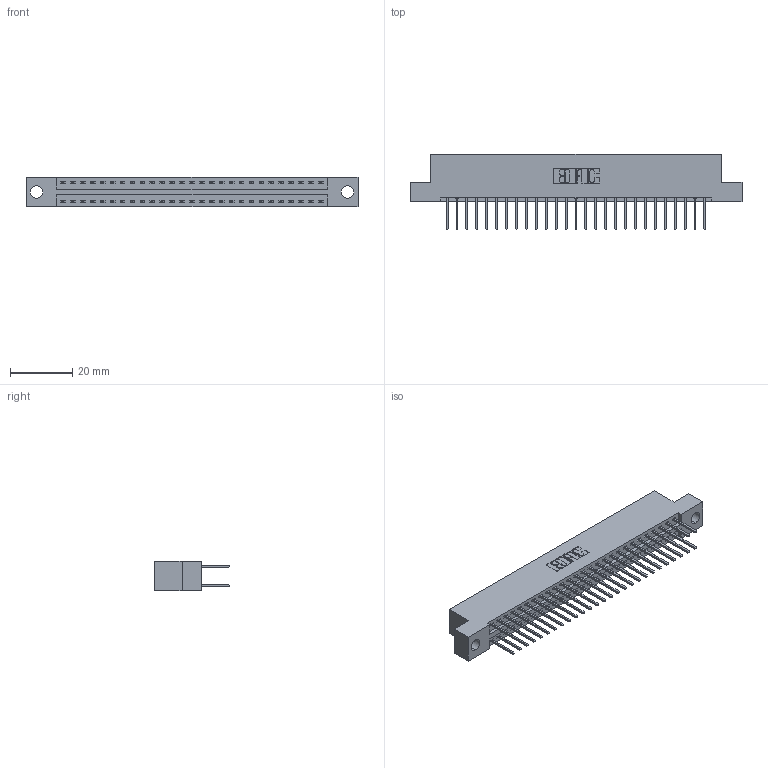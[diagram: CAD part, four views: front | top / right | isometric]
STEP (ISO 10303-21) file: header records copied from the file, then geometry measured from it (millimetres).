
FILE_DESCRIPTION (( 'STEP AP203' ), '1' );
FILE_NAME ('396-054-526-204.STEP', '2019-10-30T14:17:34', ( '' ), ( '' ), 'SwSTEP 2.0', 'SolidWorks 2016', '' );
FILE_SCHEMA (( 'CONFIG_CONTROL_DESIGN' ));
Length unit declared in the file: inch
Products named in the file (3): 396-054-526-204; 346 Part_Flush Mounting Lugs - 0.156 Dia-TH; 345-292-001_345-293-126
Assembly tree (55 placements, depth 2):
  396-054-526-204
    346 Part_Flush Mounting Lugs - 0.156 Dia-TH
    345-292-001_345-293-126  x54
Bounding box: 106.3 x 24.13 x 9.4 mm (x, y, z)
Volume: 10249.7 mm3; surface area: 14062.8 mm2
Topology: 55 solids, 55 shells, 2930 faces, 8699 edges, 5726 vertices
Faces by surface type: plane 1966, cylinder 964
Entity records: 19661 total; most frequent: CARTESIAN_POINT 3260, ORIENTED_EDGE 3194, DIRECTION 2925, EDGE_CURVE 1597, VECTOR 1357, LINE 1357, VERTEX_POINT 1062, AXIS2_PLACEMENT_3D 784
